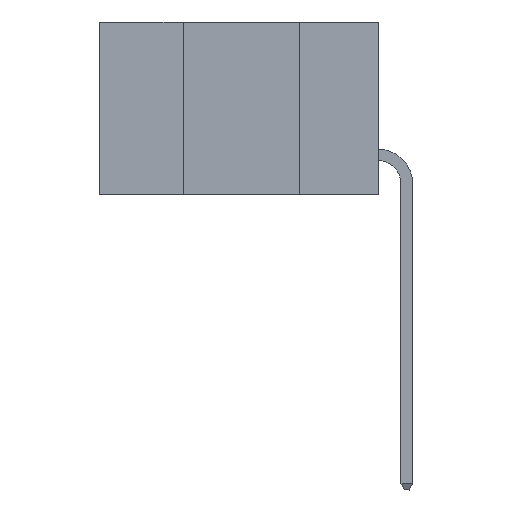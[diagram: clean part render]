
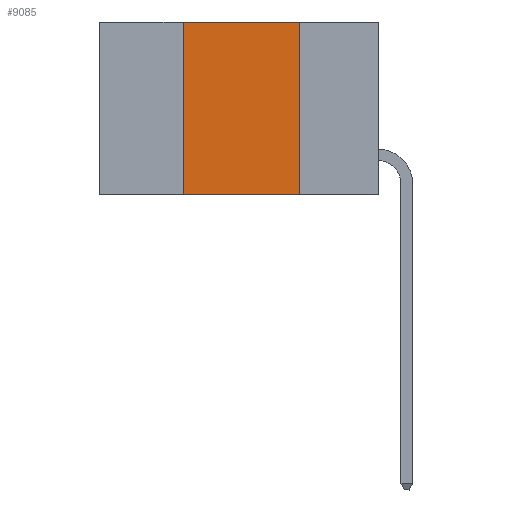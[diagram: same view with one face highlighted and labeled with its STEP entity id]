
A CAD part, left-side view. The second image highlights one B-rep face of the part: STEP entity #9085.
In plain terms, the highlighted planar face has unit normal (-1, 0, 0).
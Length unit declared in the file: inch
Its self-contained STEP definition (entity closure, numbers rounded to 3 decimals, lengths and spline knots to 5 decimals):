
#256 = CARTESIAN_POINT ( 'NONE',  ( 0., 0.17, -0.37 ) ) ;
#829 = DIRECTION ( 'NONE',  ( 0., 0., -1. ) ) ;
#990 = ORIENTED_EDGE ( 'NONE', *, *, #4030, .T. ) ;
#1719 = VECTOR ( 'NONE', #6367, 39.37008 ) ;
#2869 = CARTESIAN_POINT ( 'NONE',  ( 0., 0.42, -0.37 ) ) ;
#3131 = VECTOR ( 'NONE', #8486, 39.37008 ) ;
#3221 = EDGE_LOOP ( 'NONE', ( #11493, #11896, #3352, #990 ) ) ;
#3352 = ORIENTED_EDGE ( 'NONE', *, *, #9457, .F. ) ;
#3709 = LINE ( 'NONE', #9788, #6856 ) ;
#3866 = LINE ( 'NONE', #2869, #9597 ) ;
#3885 = DIRECTION ( 'NONE',  ( 1., 0., 0. ) ) ;
#3944 = EDGE_CURVE ( 'NONE', #12486, #11351, #8223, .T. ) ;
#4030 = EDGE_CURVE ( 'NONE', #6434, #11351, #5418, .T. ) ;
#4920 = DIRECTION ( 'NONE',  ( 0., -1., 0. ) ) ;
#5418 = LINE ( 'NONE', #12178, #1719 ) ;
#5799 = DIRECTION ( 'NONE',  ( 0., 0., 1. ) ) ;
#6020 = VERTEX_POINT ( 'NONE', #10717 ) ;
#6367 = DIRECTION ( 'NONE',  ( 0., -1., 0. ) ) ;
#6434 = VERTEX_POINT ( 'NONE', #8575 ) ;
#6495 = EDGE_CURVE ( 'NONE', #6020, #12486, #3709, .T. ) ;
#6856 = VECTOR ( 'NONE', #4920, 39.37008 ) ;
#8223 = LINE ( 'NONE', #10421, #3131 ) ;
#8486 = DIRECTION ( 'NONE',  ( 0., 0., -1. ) ) ;
#8575 = CARTESIAN_POINT ( 'NONE',  ( 0., 0.42, -0.37 ) ) ;
#8685 = FACE_OUTER_BOUND ( 'NONE', #3221, .T. ) ;
#9085 = ADVANCED_FACE ( 'NONE', ( #8685 ), #11619, .F. ) ;
#9457 = EDGE_CURVE ( 'NONE', #6434, #6020, #3866, .T. ) ;
#9597 = VECTOR ( 'NONE', #5799, 39.37008 ) ;
#9788 = CARTESIAN_POINT ( 'NONE',  ( 0., 0.6, 0. ) ) ;
#10421 = CARTESIAN_POINT ( 'NONE',  ( 0., 0.17, -0.37 ) ) ;
#10717 = CARTESIAN_POINT ( 'NONE',  ( 0., 0.42, 0. ) ) ;
#10837 = AXIS2_PLACEMENT_3D ( 'NONE', #12629, #3885, #829 ) ;
#11351 = VERTEX_POINT ( 'NONE', #256 ) ;
#11493 = ORIENTED_EDGE ( 'NONE', *, *, #3944, .F. ) ;
#11619 = PLANE ( 'NONE',  #10837 ) ;
#11805 = CARTESIAN_POINT ( 'NONE',  ( 0., 0.17, 0. ) ) ;
#11896 = ORIENTED_EDGE ( 'NONE', *, *, #6495, .F. ) ;
#12178 = CARTESIAN_POINT ( 'NONE',  ( 0., 0.6, -0.37 ) ) ;
#12486 = VERTEX_POINT ( 'NONE', #11805 ) ;
#12629 = CARTESIAN_POINT ( 'NONE',  ( 0., 0.6, 0. ) ) ;
